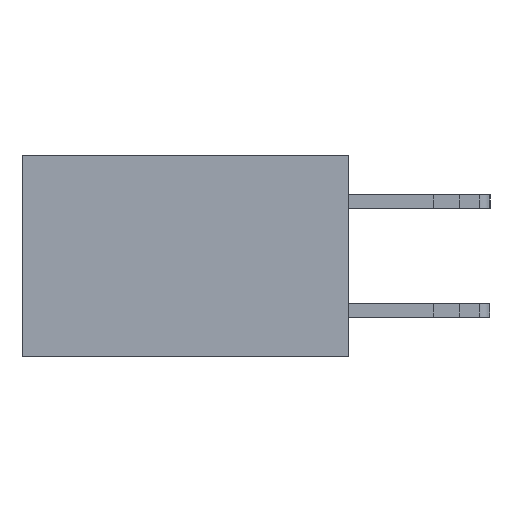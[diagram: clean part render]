
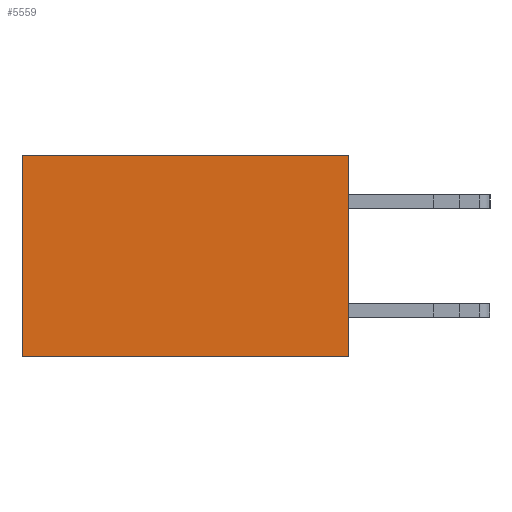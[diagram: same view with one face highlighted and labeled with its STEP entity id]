
A CAD part, left-side view. The second image highlights one B-rep face of the part: STEP entity #5559.
In plain terms, the highlighted planar face has unit normal (-1, 0, 0).
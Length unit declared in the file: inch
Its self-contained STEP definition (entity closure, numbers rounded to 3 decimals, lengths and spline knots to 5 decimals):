
#2 = PLANE ( 'NONE',  #10402 ) ;
#1386 = VECTOR ( 'NONE', #15704, 39.37008 ) ;
#1882 = ORIENTED_EDGE ( 'NONE', *, *, #5823, .F. ) ;
#2659 = VECTOR ( 'NONE', #21675, 39.37008 ) ;
#2865 = VERTEX_POINT ( 'NONE', #11984 ) ;
#3907 = VERTEX_POINT ( 'NONE', #20702 ) ;
#4522 = CARTESIAN_POINT ( 'NONE',  ( 0.298, 0., 0. ) ) ;
#5292 = EDGE_LOOP ( 'NONE', ( #7721, #1882, #15315, #21667 ) ) ;
#5559 = ADVANCED_FACE ( 'NONE', ( #15075 ), #2, .F. ) ;
#5823 = EDGE_CURVE ( 'NONE', #15609, #3907, #9704, .T. ) ;
#6390 = CARTESIAN_POINT ( 'NONE',  ( 0.298, 0.6, 0. ) ) ;
#6413 = DIRECTION ( 'NONE',  ( 0., 0., -1. ) ) ;
#6470 = CARTESIAN_POINT ( 'NONE',  ( 0.298, 0., 0. ) ) ;
#7612 = EDGE_CURVE ( 'NONE', #2865, #3907, #18744, .T. ) ;
#7678 = LINE ( 'NONE', #6470, #2659 ) ;
#7721 = ORIENTED_EDGE ( 'NONE', *, *, #7612, .T. ) ;
#9704 = LINE ( 'NONE', #15173, #18207 ) ;
#10402 = AXIS2_PLACEMENT_3D ( 'NONE', #4522, #17893, #19592 ) ;
#11460 = EDGE_CURVE ( 'NONE', #15867, #2865, #14400, .T. ) ;
#11984 = CARTESIAN_POINT ( 'NONE',  ( 0.298, 0.6, 0. ) ) ;
#13681 = EDGE_CURVE ( 'NONE', #15867, #15609, #7678, .T. ) ;
#13977 = CARTESIAN_POINT ( 'NONE',  ( 0.298, 0., 0. ) ) ;
#14282 = VECTOR ( 'NONE', #6413, 39.37008 ) ;
#14400 = LINE ( 'NONE', #13977, #1386 ) ;
#15075 = FACE_OUTER_BOUND ( 'NONE', #5292, .T. ) ;
#15173 = CARTESIAN_POINT ( 'NONE',  ( 0.298, 0., -0.37 ) ) ;
#15315 = ORIENTED_EDGE ( 'NONE', *, *, #13681, .F. ) ;
#15609 = VERTEX_POINT ( 'NONE', #20562 ) ;
#15704 = DIRECTION ( 'NONE',  ( 0., 1., 0. ) ) ;
#15867 = VERTEX_POINT ( 'NONE', #16213 ) ;
#16213 = CARTESIAN_POINT ( 'NONE',  ( 0.298, 0., 0. ) ) ;
#17893 = DIRECTION ( 'NONE',  ( 1., 0., 0. ) ) ;
#18207 = VECTOR ( 'NONE', #19851, 39.37008 ) ;
#18744 = LINE ( 'NONE', #6390, #14282 ) ;
#19592 = DIRECTION ( 'NONE',  ( 0., 0., -1. ) ) ;
#19851 = DIRECTION ( 'NONE',  ( 0., 1., 0. ) ) ;
#20562 = CARTESIAN_POINT ( 'NONE',  ( 0.298, 0., -0.37 ) ) ;
#20702 = CARTESIAN_POINT ( 'NONE',  ( 0.298, 0.6, -0.37 ) ) ;
#21667 = ORIENTED_EDGE ( 'NONE', *, *, #11460, .T. ) ;
#21675 = DIRECTION ( 'NONE',  ( 0., 0., -1. ) ) ;
